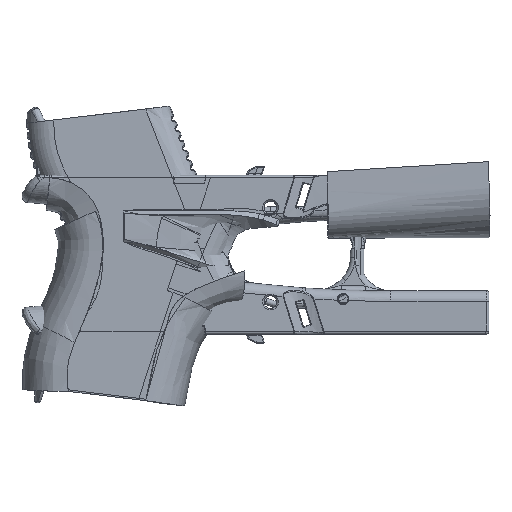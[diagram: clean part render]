
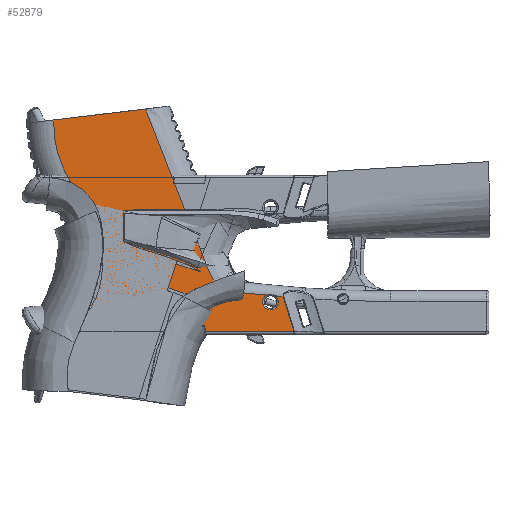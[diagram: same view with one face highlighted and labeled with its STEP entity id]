
A CAD part, front view. The second image highlights one B-rep face of the part: STEP entity #52879.
In plain terms, the highlighted planar face has unit normal (0, -1, 0).
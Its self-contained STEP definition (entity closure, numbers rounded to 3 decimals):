
#2415=CIRCLE('',#62670,35.645);
#2416=CIRCLE('',#62672,2.625);
#2417=CIRCLE('',#62673,156.771);
#2418=CIRCLE('',#62674,0.45);
#2419=CIRCLE('',#62675,0.45);
#2420=CIRCLE('',#62676,77.599);
#2421=CIRCLE('',#62677,27.167);
#2422=CIRCLE('',#62678,18.891);
#2423=CIRCLE('',#62679,0.8);
#4718=LINE('',#101035,#7281);
#4719=LINE('',#101038,#7282);
#4720=LINE('',#101040,#7283);
#4721=LINE('',#101044,#7284);
#4722=LINE('',#101048,#7285);
#4723=LINE('',#101055,#7286);
#4724=LINE('',#101059,#7287);
#4725=LINE('',#101063,#7288);
#4726=LINE('',#101065,#7289);
#4727=LINE('',#101067,#7290);
#4728=LINE('',#101074,#7291);
#4729=LINE('',#101076,#7292);
#4730=LINE('',#101080,#7293);
#4731=LINE('',#101082,#7294);
#4732=LINE('',#101084,#7295);
#4733=LINE('',#101086,#7296);
#4734=LINE('',#101088,#7297);
#7281=VECTOR('',#69256,1000.);
#7282=VECTOR('',#69257,1000.);
#7283=VECTOR('',#69258,1000.);
#7284=VECTOR('',#69261,1000.);
#7285=VECTOR('',#69264,1000.);
#7286=VECTOR('',#69265,1000.);
#7287=VECTOR('',#69268,1000.);
#7288=VECTOR('',#69271,1000.);
#7289=VECTOR('',#69272,1000.);
#7290=VECTOR('',#69273,1000.);
#7291=VECTOR('',#69280,1000.);
#7292=VECTOR('',#69281,1000.);
#7293=VECTOR('',#69284,1000.);
#7294=VECTOR('',#69285,1000.);
#7295=VECTOR('',#69286,1000.);
#7296=VECTOR('',#69287,1000.);
#7297=VECTOR('',#69288,1000.);
#9237=PLANE('',#62671);
#15415=ORIENTED_EDGE('',*,*,#29527,.F.);
#15416=ORIENTED_EDGE('',*,*,#29528,.F.);
#15417=ORIENTED_EDGE('',*,*,#29529,.F.);
#15418=ORIENTED_EDGE('',*,*,#29530,.F.);
#15419=ORIENTED_EDGE('',*,*,#29531,.F.);
#15420=ORIENTED_EDGE('',*,*,#29532,.F.);
#15421=ORIENTED_EDGE('',*,*,#29533,.T.);
#15422=ORIENTED_EDGE('',*,*,#29534,.F.);
#15423=ORIENTED_EDGE('',*,*,#29535,.F.);
#15424=ORIENTED_EDGE('',*,*,#29536,.F.);
#15425=ORIENTED_EDGE('',*,*,#29537,.F.);
#15426=ORIENTED_EDGE('',*,*,#29538,.F.);
#15427=ORIENTED_EDGE('',*,*,#29539,.F.);
#15428=ORIENTED_EDGE('',*,*,#29540,.T.);
#15429=ORIENTED_EDGE('',*,*,#29541,.F.);
#15430=ORIENTED_EDGE('',*,*,#29526,.F.);
#15431=ORIENTED_EDGE('',*,*,#29542,.F.);
#15432=ORIENTED_EDGE('',*,*,#29543,.F.);
#15433=ORIENTED_EDGE('',*,*,#29544,.F.);
#15434=ORIENTED_EDGE('',*,*,#29545,.F.);
#15435=ORIENTED_EDGE('',*,*,#29546,.F.);
#15436=ORIENTED_EDGE('',*,*,#29547,.F.);
#15437=ORIENTED_EDGE('',*,*,#29548,.F.);
#15438=ORIENTED_EDGE('',*,*,#29549,.F.);
#15439=ORIENTED_EDGE('',*,*,#29550,.F.);
#15440=ORIENTED_EDGE('',*,*,#29551,.F.);
#15441=ORIENTED_EDGE('',*,*,#29552,.F.);
#29526=EDGE_CURVE('',#36886,#36853,#2415,.T.);
#29527=EDGE_CURVE('',#36887,#36888,#4718,.T.);
#29528=EDGE_CURVE('',#36889,#36887,#4719,.T.);
#29529=EDGE_CURVE('',#36890,#36889,#4720,.T.);
#29530=EDGE_CURVE('',#36891,#36890,#2416,.T.);
#29531=EDGE_CURVE('',#36892,#36891,#4721,.T.);
#29532=EDGE_CURVE('',#36893,#36892,#2417,.T.);
#29533=EDGE_CURVE('',#36893,#36894,#4722,.T.);
#29534=EDGE_CURVE('',#36895,#36894,#41498,.T.);
#29535=EDGE_CURVE('',#36896,#36895,#4723,.T.);
#29536=EDGE_CURVE('',#36897,#36896,#2418,.T.);
#29537=EDGE_CURVE('',#36898,#36897,#4724,.T.);
#29538=EDGE_CURVE('',#36899,#36898,#2419,.T.);
#29539=EDGE_CURVE('',#36900,#36899,#4725,.T.);
#29540=EDGE_CURVE('',#36900,#36901,#4726,.T.);
#29541=EDGE_CURVE('',#36853,#36901,#4727,.T.);
#29542=EDGE_CURVE('',#36902,#36886,#2420,.T.);
#29543=EDGE_CURVE('',#36903,#36902,#2421,.T.);
#29544=EDGE_CURVE('',#36904,#36903,#2422,.T.);
#29545=EDGE_CURVE('',#36905,#36904,#4728,.T.);
#29546=EDGE_CURVE('',#36906,#36905,#4729,.T.);
#29547=EDGE_CURVE('',#36907,#36906,#2423,.T.);
#29548=EDGE_CURVE('',#36908,#36907,#4730,.T.);
#29549=EDGE_CURVE('',#36909,#36908,#4731,.T.);
#29550=EDGE_CURVE('',#36910,#36909,#4732,.T.);
#29551=EDGE_CURVE('',#36911,#36910,#4733,.T.);
#29552=EDGE_CURVE('',#36888,#36911,#4734,.T.);
#36853=VERTEX_POINT('',#100775);
#36886=VERTEX_POINT('',#101032);
#36887=VERTEX_POINT('',#101036);
#36888=VERTEX_POINT('',#101037);
#36889=VERTEX_POINT('',#101039);
#36890=VERTEX_POINT('',#101041);
#36891=VERTEX_POINT('',#101043);
#36892=VERTEX_POINT('',#101045);
#36893=VERTEX_POINT('',#101047);
#36894=VERTEX_POINT('',#101049);
#36895=VERTEX_POINT('',#101054);
#36896=VERTEX_POINT('',#101056);
#36897=VERTEX_POINT('',#101058);
#36898=VERTEX_POINT('',#101060);
#36899=VERTEX_POINT('',#101062);
#36900=VERTEX_POINT('',#101064);
#36901=VERTEX_POINT('',#101066);
#36902=VERTEX_POINT('',#101069);
#36903=VERTEX_POINT('',#101071);
#36904=VERTEX_POINT('',#101073);
#36905=VERTEX_POINT('',#101075);
#36906=VERTEX_POINT('',#101077);
#36907=VERTEX_POINT('',#101079);
#36908=VERTEX_POINT('',#101081);
#36909=VERTEX_POINT('',#101083);
#36910=VERTEX_POINT('',#101085);
#36911=VERTEX_POINT('',#101087);
#41498=B_SPLINE_CURVE_WITH_KNOTS('',3,(#101050,#101051,#101052,#101053),
 .UNSPECIFIED.,.F.,.F.,(4,4),(-0.106,-0.092),
 .UNSPECIFIED.);
#45032=EDGE_LOOP('',(#15415,#15416,#15417,#15418,#15419,#15420,#15421,#15422,
#15423,#15424,#15425,#15426,#15427,#15428,#15429,#15430,#15431,#15432,#15433,
#15434,#15435,#15436,#15437,#15438,#15439,#15440,#15441));
#48471=FACE_BOUND('',#45032,.T.);
#52879=ADVANCED_FACE('',(#48471),#9237,.F.);
#62670=AXIS2_PLACEMENT_3D('',#101033,#69252,#69253);
#62671=AXIS2_PLACEMENT_3D('',#101034,#69254,#69255);
#62672=AXIS2_PLACEMENT_3D('',#101042,#69259,#69260);
#62673=AXIS2_PLACEMENT_3D('',#101046,#69262,#69263);
#62674=AXIS2_PLACEMENT_3D('',#101057,#69266,#69267);
#62675=AXIS2_PLACEMENT_3D('',#101061,#69269,#69270);
#62676=AXIS2_PLACEMENT_3D('',#101068,#69274,#69275);
#62677=AXIS2_PLACEMENT_3D('',#101070,#69276,#69277);
#62678=AXIS2_PLACEMENT_3D('',#101072,#69278,#69279);
#62679=AXIS2_PLACEMENT_3D('',#101078,#69282,#69283);
#69252=DIRECTION('',(0.,1.,0.));
#69253=DIRECTION('',(-0.961,0.,-0.276));
#69254=DIRECTION('',(0.,1.,0.));
#69255=DIRECTION('',(1.,0.,0.));
#69256=DIRECTION('',(-1.,0.,0.));
#69257=DIRECTION('',(0.292,0.,-0.956));
#69258=DIRECTION('',(0.996,0.,-0.092));
#69259=DIRECTION('',(0.,-1.,0.));
#69260=DIRECTION('',(-1.,0.,0.));
#69261=DIRECTION('',(0.996,0.,-0.092));
#69262=DIRECTION('',(0.,-1.,0.));
#69263=DIRECTION('',(-0.937,0.,-0.35));
#69264=DIRECTION('',(-0.363,0.,0.932));
#69265=DIRECTION('',(0.951,0.,0.309));
#69266=DIRECTION('',(0.,-1.,0.));
#69267=DIRECTION('',(-0.454,0.,-0.891));
#69268=DIRECTION('',(0.309,0.,-0.951));
#69269=DIRECTION('',(0.,-1.,0.));
#69270=DIRECTION('',(-0.891,0.,0.454));
#69271=DIRECTION('',(-0.951,0.,-0.309));
#69272=DIRECTION('',(-0.363,0.,0.932));
#69273=DIRECTION('',(0.993,0.,0.119));
#69274=DIRECTION('',(0.,-1.,0.));
#69275=DIRECTION('',(0.907,0.,0.421));
#69276=DIRECTION('',(0.,-1.,0.));
#69277=DIRECTION('',(0.998,0.,-0.06));
#69278=DIRECTION('',(0.,-1.,0.));
#69279=DIRECTION('',(0.592,0.,-0.806));
#69280=DIRECTION('',(-1.,0.,0.));
#69281=DIRECTION('',(0.,0.,-1.));
#69282=DIRECTION('',(0.,-1.,0.));
#69283=DIRECTION('',(-0.707,0.,0.707));
#69284=DIRECTION('',(0.,0.,-1.));
#69285=DIRECTION('',(-1.,0.,0.));
#69286=DIRECTION('',(0.,0.,1.));
#69287=DIRECTION('',(-1.,0.,0.));
#69288=DIRECTION('',(0.,0.,1.));
#100775=CARTESIAN_POINT('',(-68.982,-11.5,45.003));
#101032=CARTESIAN_POINT('',(-63.213,-11.5,24.169));
#101033=CARTESIAN_POINT('',(-33.363,-11.5,43.651));
#101034=CARTESIAN_POINT('',(-1.777,-11.5,10.863));
#101035=CARTESIAN_POINT('',(37.236,-11.5,-25.75));
#101036=CARTESIAN_POINT('',(11.185,-11.5,-25.75));
#101037=CARTESIAN_POINT('',(-18.45,-11.5,-25.75));
#101038=CARTESIAN_POINT('',(5.553,-11.5,-7.328));
#101039=CARTESIAN_POINT('',(7.57,-11.5,-13.924));
#101040=CARTESIAN_POINT('',(4.861,-11.5,-13.675));
#101041=CARTESIAN_POINT('',(4.906,-11.5,-13.679));
#101042=CARTESIAN_POINT('',(3.343,-11.5,-15.788));
#101043=CARTESIAN_POINT('',(2.19,-11.5,-13.43));
#101044=CARTESIAN_POINT('',(4.861,-11.5,-13.675));
#101045=CARTESIAN_POINT('',(-14.141,-11.5,-11.929));
#101046=CARTESIAN_POINT('',(126.663,-11.5,57.001));
#101047=CARTESIAN_POINT('',(-20.166,-11.5,2.06));
#101048=CARTESIAN_POINT('',(-37.545,-11.5,46.678));
#101049=CARTESIAN_POINT('',(-21.075,-11.5,4.396));
#101050=CARTESIAN_POINT('',(-21.284,-11.5,4.253));
#101051=CARTESIAN_POINT('',(-21.203,-11.5,4.28));
#101052=CARTESIAN_POINT('',(-21.129,-11.5,4.33));
#101053=CARTESIAN_POINT('',(-21.075,-11.5,4.396));
#101054=CARTESIAN_POINT('',(-21.284,-11.5,4.253));
#101055=CARTESIAN_POINT('',(-11.372,-11.5,7.474));
#101056=CARTESIAN_POINT('',(-27.466,-11.5,2.245));
#101057=CARTESIAN_POINT('',(-27.605,-11.5,2.673));
#101058=CARTESIAN_POINT('',(-28.033,-11.5,2.534));
#101059=CARTESIAN_POINT('',(-28.119,-11.5,2.799));
#101060=CARTESIAN_POINT('',(-30.659,-11.5,10.618));
#101061=CARTESIAN_POINT('',(-30.231,-11.5,10.757));
#101062=CARTESIAN_POINT('',(-30.37,-11.5,11.185));
#101063=CARTESIAN_POINT('',(-17.605,-11.5,15.332));
#101064=CARTESIAN_POINT('',(-24.467,-11.5,13.103));
#101065=CARTESIAN_POINT('',(-37.545,-11.5,46.678));
#101066=CARTESIAN_POINT('',(-38.322,-11.5,48.672));
#101067=CARTESIAN_POINT('',(-6.737,-11.5,52.452));
#101068=CARTESIAN_POINT('',(-128.196,-11.5,-18.243));
#101069=CARTESIAN_POINT('',(-53.881,-11.5,4.09));
#101070=CARTESIAN_POINT('',(-79.899,-11.5,-3.729));
#101071=CARTESIAN_POINT('',(-55.002,-11.5,-14.602));
#101072=CARTESIAN_POINT('',(-72.315,-11.5,-7.041));
#101073=CARTESIAN_POINT('',(-69.695,-11.5,-25.75));
#101074=CARTESIAN_POINT('',(37.236,-11.5,-25.75));
#101075=CARTESIAN_POINT('',(-29.05,-11.5,-25.75));
#101076=CARTESIAN_POINT('',(-29.05,-11.5,-7.056));
#101077=CARTESIAN_POINT('',(-29.05,-11.5,-25.475));
#101078=CARTESIAN_POINT('',(-28.25,-11.5,-25.475));
#101079=CARTESIAN_POINT('',(-28.98,-11.5,-25.148));
#101080=CARTESIAN_POINT('',(-28.98,-11.5,-7.056));
#101081=CARTESIAN_POINT('',(-28.98,-11.5,-23.745));
#101082=CARTESIAN_POINT('',(-10.264,-11.5,-23.745));
#101083=CARTESIAN_POINT('',(-18.52,-11.5,-23.745));
#101084=CARTESIAN_POINT('',(-18.52,-11.5,-7.056));
#101085=CARTESIAN_POINT('',(-18.52,-11.5,-24.675));
#101086=CARTESIAN_POINT('',(-10.264,-11.5,-24.675));
#101087=CARTESIAN_POINT('',(-18.45,-11.5,-24.675));
#101088=CARTESIAN_POINT('',(-18.45,-11.5,-7.818));
